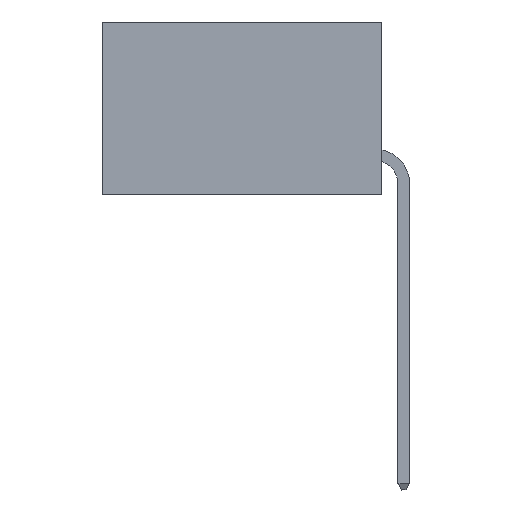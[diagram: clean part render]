
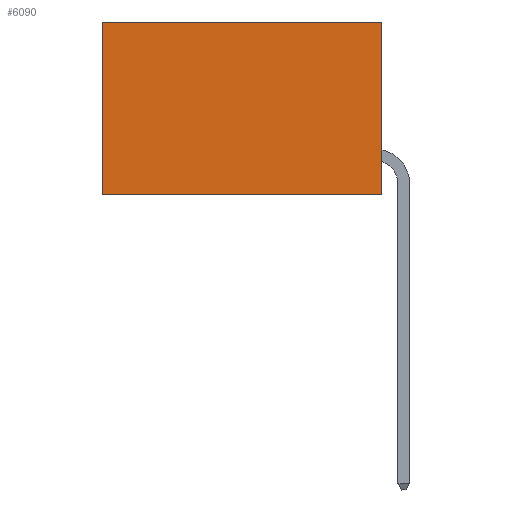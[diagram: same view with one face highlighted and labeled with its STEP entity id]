
A CAD part, left-side view. The second image highlights one B-rep face of the part: STEP entity #6090.
In plain terms, the highlighted planar face has unit normal (-1, 0, 0).
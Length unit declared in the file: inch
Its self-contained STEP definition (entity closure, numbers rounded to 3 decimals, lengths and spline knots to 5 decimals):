
#188 = DIRECTION ( 'NONE',  ( 0., 0., -1. ) ) ;
#1694 = PLANE ( 'NONE',  #11495 ) ;
#1724 = EDGE_LOOP ( 'NONE', ( #20231, #19331, #4007, #2264 ) ) ;
#2226 = CARTESIAN_POINT ( 'NONE',  ( 0.2875, 0.6, 0. ) ) ;
#2264 = ORIENTED_EDGE ( 'NONE', *, *, #7466, .T. ) ;
#2538 = DIRECTION ( 'NONE',  ( 0., 1., 0. ) ) ;
#2632 = VECTOR ( 'NONE', #8452, 39.37008 ) ;
#2695 = FACE_OUTER_BOUND ( 'NONE', #1724, .T. ) ;
#3369 = VERTEX_POINT ( 'NONE', #7665 ) ;
#3521 = EDGE_CURVE ( 'NONE', #4298, #3369, #5873, .T. ) ;
#4007 = ORIENTED_EDGE ( 'NONE', *, *, #10113, .F. ) ;
#4298 = VERTEX_POINT ( 'NONE', #12107 ) ;
#5014 = CARTESIAN_POINT ( 'NONE',  ( 0.2875, 0., 0. ) ) ;
#5035 = DIRECTION ( 'NONE',  ( 1., 0., 0. ) ) ;
#5582 = VECTOR ( 'NONE', #188, 39.37008 ) ;
#5690 = VERTEX_POINT ( 'NONE', #8571 ) ;
#5873 = LINE ( 'NONE', #10532, #20721 ) ;
#6090 = ADVANCED_FACE ( 'NONE', ( #2695 ), #1694, .F. ) ;
#7218 = DIRECTION ( 'NONE',  ( 0., 0., -1. ) ) ;
#7466 = EDGE_CURVE ( 'NONE', #10494, #5690, #14503, .T. ) ;
#7629 = LINE ( 'NONE', #13153, #5582 ) ;
#7665 = CARTESIAN_POINT ( 'NONE',  ( 0.2875, 0.6, -0.37 ) ) ;
#8452 = DIRECTION ( 'NONE',  ( 0., 1., 0. ) ) ;
#8571 = CARTESIAN_POINT ( 'NONE',  ( 0.2875, 0.6, 0. ) ) ;
#8933 = EDGE_CURVE ( 'NONE', #5690, #3369, #18938, .T. ) ;
#9691 = DIRECTION ( 'NONE',  ( 0., 0., -1. ) ) ;
#10113 = EDGE_CURVE ( 'NONE', #10494, #4298, #7629, .T. ) ;
#10494 = VERTEX_POINT ( 'NONE', #5014 ) ;
#10532 = CARTESIAN_POINT ( 'NONE',  ( 0.2875, 0., -0.37 ) ) ;
#11495 = AXIS2_PLACEMENT_3D ( 'NONE', #16449, #5035, #9691 ) ;
#12107 = CARTESIAN_POINT ( 'NONE',  ( 0.2875, 0., -0.37 ) ) ;
#13153 = CARTESIAN_POINT ( 'NONE',  ( 0.2875, 0., 0. ) ) ;
#13287 = CARTESIAN_POINT ( 'NONE',  ( 0.2875, 0., 0. ) ) ;
#14503 = LINE ( 'NONE', #13287, #2632 ) ;
#14924 = VECTOR ( 'NONE', #7218, 39.37008 ) ;
#16449 = CARTESIAN_POINT ( 'NONE',  ( 0.2875, 0., 0. ) ) ;
#18938 = LINE ( 'NONE', #2226, #14924 ) ;
#19331 = ORIENTED_EDGE ( 'NONE', *, *, #3521, .F. ) ;
#20231 = ORIENTED_EDGE ( 'NONE', *, *, #8933, .T. ) ;
#20721 = VECTOR ( 'NONE', #2538, 39.37008 ) ;
